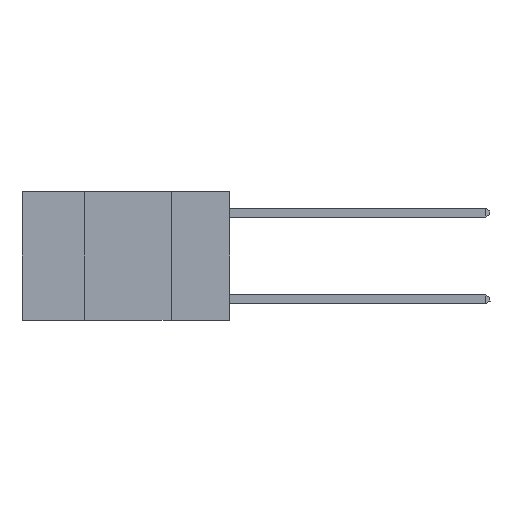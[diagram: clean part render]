
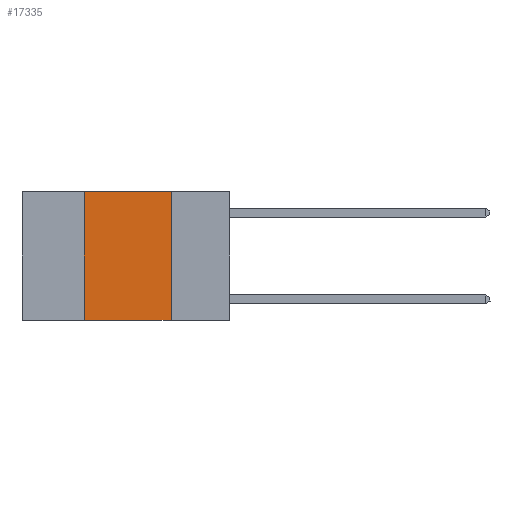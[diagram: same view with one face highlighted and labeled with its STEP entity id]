
A CAD part, left-side view. The second image highlights one B-rep face of the part: STEP entity #17335.
In plain terms, the highlighted planar face has unit normal (-1, 0, 0).
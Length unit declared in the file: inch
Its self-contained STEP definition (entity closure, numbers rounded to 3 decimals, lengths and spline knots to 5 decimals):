
#117 = VECTOR ( 'NONE', #17028, 39.37008 ) ;
#1171 = AXIS2_PLACEMENT_3D ( 'NONE', #1610, #13646, #3329 ) ;
#1392 = CARTESIAN_POINT ( 'NONE',  ( 0., 0.42, 0. ) ) ;
#1610 = CARTESIAN_POINT ( 'NONE',  ( 0., 0.6, 0. ) ) ;
#2413 = VECTOR ( 'NONE', #17485, 39.37008 ) ;
#2469 = FACE_OUTER_BOUND ( 'NONE', #14614, .T. ) ;
#2796 = VECTOR ( 'NONE', #21780, 39.37008 ) ;
#3329 = DIRECTION ( 'NONE',  ( 0., 0., -1. ) ) ;
#3352 = EDGE_CURVE ( 'NONE', #5263, #8102, #19402, .T. ) ;
#3520 = CARTESIAN_POINT ( 'NONE',  ( 0., 0.42, -0.37 ) ) ;
#3599 = ORIENTED_EDGE ( 'NONE', *, *, #6840, .F. ) ;
#4495 = EDGE_CURVE ( 'NONE', #5263, #11349, #16488, .T. ) ;
#5244 = VECTOR ( 'NONE', #9034, 39.37008 ) ;
#5263 = VERTEX_POINT ( 'NONE', #3520 ) ;
#6840 = EDGE_CURVE ( 'NONE', #7170, #8102, #11590, .T. ) ;
#7170 = VERTEX_POINT ( 'NONE', #14843 ) ;
#7249 = CARTESIAN_POINT ( 'NONE',  ( 0., 0.17, 0. ) ) ;
#8102 = VERTEX_POINT ( 'NONE', #20554 ) ;
#8470 = PLANE ( 'NONE',  #1171 ) ;
#8744 = ORIENTED_EDGE ( 'NONE', *, *, #4495, .F. ) ;
#9034 = DIRECTION ( 'NONE',  ( 0., -1., 0. ) ) ;
#9245 = LINE ( 'NONE', #20374, #117 ) ;
#10172 = EDGE_CURVE ( 'NONE', #11349, #7170, #9245, .T. ) ;
#11349 = VERTEX_POINT ( 'NONE', #13330 ) ;
#11590 = LINE ( 'NONE', #7249, #2413 ) ;
#12414 = CARTESIAN_POINT ( 'NONE',  ( 0., 0.6, -0.37 ) ) ;
#12755 = ORIENTED_EDGE ( 'NONE', *, *, #10172, .F. ) ;
#13294 = ORIENTED_EDGE ( 'NONE', *, *, #3352, .T. ) ;
#13330 = CARTESIAN_POINT ( 'NONE',  ( 0., 0.42, 0. ) ) ;
#13646 = DIRECTION ( 'NONE',  ( 1., 0., 0. ) ) ;
#14614 = EDGE_LOOP ( 'NONE', ( #3599, #12755, #8744, #13294 ) ) ;
#14843 = CARTESIAN_POINT ( 'NONE',  ( 0., 0.17, 0. ) ) ;
#16488 = LINE ( 'NONE', #1392, #2796 ) ;
#17028 = DIRECTION ( 'NONE',  ( 0., -1., 0. ) ) ;
#17335 = ADVANCED_FACE ( 'NONE', ( #2469 ), #8470, .F. ) ;
#17485 = DIRECTION ( 'NONE',  ( 0., 0., -1. ) ) ;
#19402 = LINE ( 'NONE', #12414, #5244 ) ;
#20374 = CARTESIAN_POINT ( 'NONE',  ( 0., 0.6, 0. ) ) ;
#20554 = CARTESIAN_POINT ( 'NONE',  ( 0., 0.17, -0.37 ) ) ;
#21780 = DIRECTION ( 'NONE',  ( 0., 0., 1. ) ) ;
